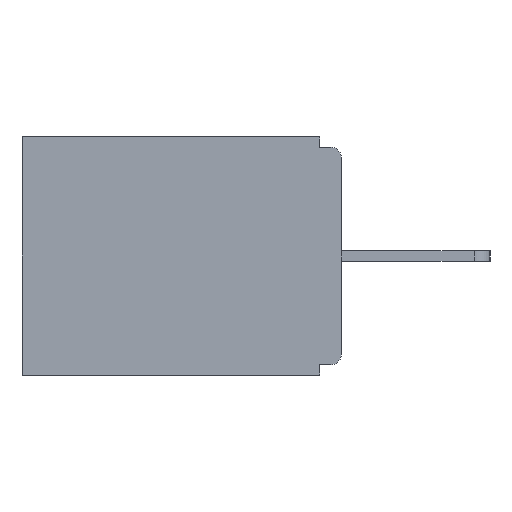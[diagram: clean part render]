
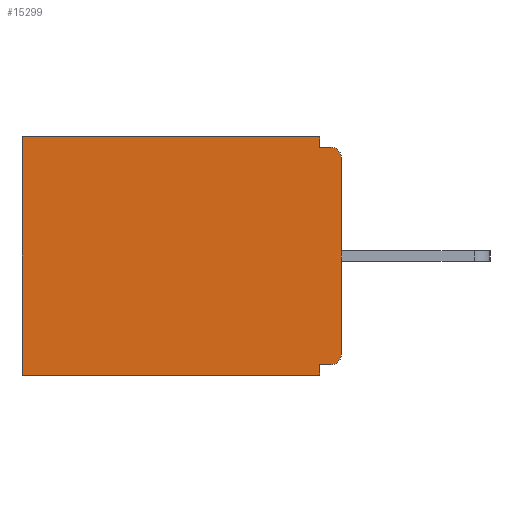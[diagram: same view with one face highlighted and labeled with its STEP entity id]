
A CAD part, left-side view. The second image highlights one B-rep face of the part: STEP entity #15299.
In plain terms, the highlighted planar face has unit normal (-1, 0, 0).
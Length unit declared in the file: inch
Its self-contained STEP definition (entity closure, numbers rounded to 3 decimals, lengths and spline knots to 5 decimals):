
#263 = DIRECTION ( 'NONE',  ( 1., 0., 0. ) ) ;
#959 = EDGE_LOOP ( 'NONE', ( #23411, #24005, #22039, #6907, #23222, #2056, #13297, #8813, #11824, #6431 ) ) ;
#1084 = LINE ( 'NONE', #23533, #19070 ) ;
#1179 = DIRECTION ( 'NONE',  ( 0., 1., 0. ) ) ;
#1988 = EDGE_CURVE ( 'NONE', #17820, #2269, #15054, .T. ) ;
#2056 = ORIENTED_EDGE ( 'NONE', *, *, #15301, .F. ) ;
#2118 = DIRECTION ( 'NONE',  ( 0., 0., -1. ) ) ;
#2269 = VERTEX_POINT ( 'NONE', #16382 ) ;
#2274 = CARTESIAN_POINT ( 'NONE',  ( 0.298, 0.46, -0.343 ) ) ;
#2517 = EDGE_CURVE ( 'NONE', #8514, #2269, #20103, .T. ) ;
#2849 = CARTESIAN_POINT ( 'NONE',  ( 0.298, 0.031, -0.015 ) ) ;
#2863 = VECTOR ( 'NONE', #7896, 39.37008 ) ;
#2955 = CARTESIAN_POINT ( 'NONE',  ( 0.298, 0.015, -0.015 ) ) ;
#3150 = CARTESIAN_POINT ( 'NONE',  ( 0.298, 0., 0. ) ) ;
#3671 = EDGE_CURVE ( 'NONE', #12043, #15829, #1084, .T. ) ;
#3954 = CARTESIAN_POINT ( 'NONE',  ( 0.298, 0.031, -0.328 ) ) ;
#4566 = EDGE_CURVE ( 'NONE', #14510, #17560, #13716, .T. ) ;
#4994 = LINE ( 'NONE', #3150, #13361 ) ;
#5144 = LINE ( 'NONE', #12687, #18317 ) ;
#5427 = EDGE_CURVE ( 'NONE', #21287, #18983, #5144, .T. ) ;
#5945 = CARTESIAN_POINT ( 'NONE',  ( 0.298, 0., 0. ) ) ;
#6192 = FACE_OUTER_BOUND ( 'NONE', #959, .T. ) ;
#6431 = ORIENTED_EDGE ( 'NONE', *, *, #1988, .F. ) ;
#6734 = CARTESIAN_POINT ( 'NONE',  ( 0.298, 0.015, -0.313 ) ) ;
#6739 = CARTESIAN_POINT ( 'NONE',  ( 0.298, 0.015, -0.328 ) ) ;
#6907 = ORIENTED_EDGE ( 'NONE', *, *, #20458, .T. ) ;
#7120 = DIRECTION ( 'NONE',  ( 0., 0., -1. ) ) ;
#7483 = AXIS2_PLACEMENT_3D ( 'NONE', #6734, #21427, #23637 ) ;
#7771 = CARTESIAN_POINT ( 'NONE',  ( 0.298, 0.031, -0.343 ) ) ;
#7790 = DIRECTION ( 'NONE',  ( 0., 1., 0. ) ) ;
#7896 = DIRECTION ( 'NONE',  ( 0., -1., 0. ) ) ;
#7973 = CARTESIAN_POINT ( 'NONE',  ( 0.298, 0.031, 0. ) ) ;
#8514 = VERTEX_POINT ( 'NONE', #6739 ) ;
#8676 = EDGE_CURVE ( 'NONE', #8514, #21287, #16363, .T. ) ;
#8813 = ORIENTED_EDGE ( 'NONE', *, *, #8676, .F. ) ;
#8965 = VECTOR ( 'NONE', #9652, 39.37008 ) ;
#9278 = CARTESIAN_POINT ( 'NONE',  ( 0.298, 0., 0. ) ) ;
#9503 = CARTESIAN_POINT ( 'NONE',  ( 0.298, 0., -0.015 ) ) ;
#9652 = DIRECTION ( 'NONE',  ( 0., 0., -1. ) ) ;
#9780 = DIRECTION ( 'NONE',  ( 0., 0., -1. ) ) ;
#10201 = CARTESIAN_POINT ( 'NONE',  ( 0.298, 0.015, -0.03 ) ) ;
#10893 = CIRCLE ( 'NONE', #20737, 0.015 ) ;
#10989 = EDGE_CURVE ( 'NONE', #17560, #11253, #15303, .T. ) ;
#11043 = DIRECTION ( 'NONE',  ( 0., 1., 0. ) ) ;
#11167 = CARTESIAN_POINT ( 'NONE',  ( 0.298, 0., -0.328 ) ) ;
#11253 = VERTEX_POINT ( 'NONE', #2955 ) ;
#11824 = ORIENTED_EDGE ( 'NONE', *, *, #2517, .T. ) ;
#11826 = DIRECTION ( 'NONE',  ( 0., 0., -1. ) ) ;
#11907 = CARTESIAN_POINT ( 'NONE',  ( 0.298, 0.46, 0. ) ) ;
#11927 = DIRECTION ( 'NONE',  ( 0., 0., -1. ) ) ;
#12043 = VERTEX_POINT ( 'NONE', #11907 ) ;
#12462 = VECTOR ( 'NONE', #9780, 39.37008 ) ;
#12687 = CARTESIAN_POINT ( 'NONE',  ( 0.298, 0.031, -0.343 ) ) ;
#13297 = ORIENTED_EDGE ( 'NONE', *, *, #5427, .F. ) ;
#13328 = CARTESIAN_POINT ( 'NONE',  ( 0.298, 0., -0.03 ) ) ;
#13361 = VECTOR ( 'NONE', #1179, 39.37008 ) ;
#13712 = CARTESIAN_POINT ( 'NONE',  ( 0.298, 0., -0.343 ) ) ;
#13716 = LINE ( 'NONE', #15318, #12462 ) ;
#14012 = AXIS2_PLACEMENT_3D ( 'NONE', #5945, #263, #2118 ) ;
#14510 = VERTEX_POINT ( 'NONE', #7973 ) ;
#15054 = LINE ( 'NONE', #9278, #8965 ) ;
#15299 = ADVANCED_FACE ( 'NONE', ( #6192 ), #20746, .F. ) ;
#15301 = EDGE_CURVE ( 'NONE', #18983, #15829, #17040, .T. ) ;
#15303 = LINE ( 'NONE', #9503, #2863 ) ;
#15318 = CARTESIAN_POINT ( 'NONE',  ( 0.298, 0.031, -0.343 ) ) ;
#15829 = VERTEX_POINT ( 'NONE', #2274 ) ;
#16363 = LINE ( 'NONE', #11167, #22931 ) ;
#16382 = CARTESIAN_POINT ( 'NONE',  ( 0.298, 0., -0.313 ) ) ;
#16575 = EDGE_CURVE ( 'NONE', #17820, #11253, #10893, .T. ) ;
#17040 = LINE ( 'NONE', #13712, #24264 ) ;
#17560 = VERTEX_POINT ( 'NONE', #2849 ) ;
#17820 = VERTEX_POINT ( 'NONE', #13328 ) ;
#18317 = VECTOR ( 'NONE', #7120, 39.37008 ) ;
#18983 = VERTEX_POINT ( 'NONE', #7771 ) ;
#19070 = VECTOR ( 'NONE', #11826, 39.37008 ) ;
#20103 = CIRCLE ( 'NONE', #7483, 0.015 ) ;
#20458 = EDGE_CURVE ( 'NONE', #14510, #12043, #4994, .T. ) ;
#20737 = AXIS2_PLACEMENT_3D ( 'NONE', #10201, #23153, #11927 ) ;
#20746 = PLANE ( 'NONE',  #14012 ) ;
#21287 = VERTEX_POINT ( 'NONE', #3954 ) ;
#21427 = DIRECTION ( 'NONE',  ( -1., 0., 0. ) ) ;
#22039 = ORIENTED_EDGE ( 'NONE', *, *, #4566, .F. ) ;
#22931 = VECTOR ( 'NONE', #11043, 39.37008 ) ;
#23153 = DIRECTION ( 'NONE',  ( -1., 0., 0. ) ) ;
#23222 = ORIENTED_EDGE ( 'NONE', *, *, #3671, .T. ) ;
#23411 = ORIENTED_EDGE ( 'NONE', *, *, #16575, .T. ) ;
#23533 = CARTESIAN_POINT ( 'NONE',  ( 0.298, 0.46, 0. ) ) ;
#23637 = DIRECTION ( 'NONE',  ( 0., 0., -1. ) ) ;
#24005 = ORIENTED_EDGE ( 'NONE', *, *, #10989, .F. ) ;
#24264 = VECTOR ( 'NONE', #7790, 39.37008 ) ;
